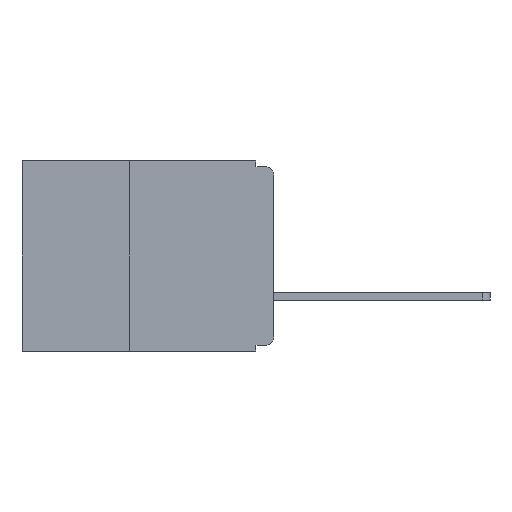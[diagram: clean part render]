
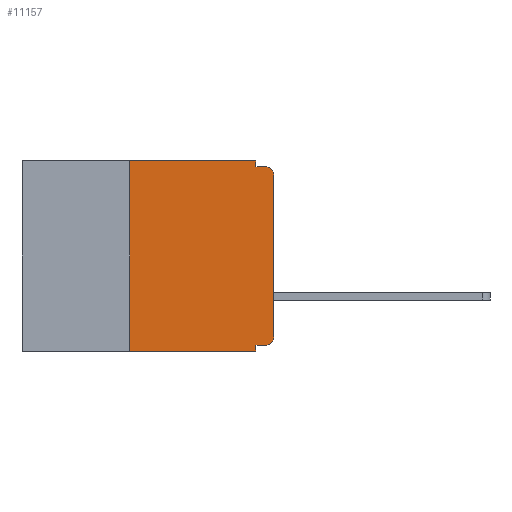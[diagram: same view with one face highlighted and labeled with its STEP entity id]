
A CAD part, left-side view. The second image highlights one B-rep face of the part: STEP entity #11157.
In plain terms, the highlighted planar face has unit normal (-1, 0, 0).
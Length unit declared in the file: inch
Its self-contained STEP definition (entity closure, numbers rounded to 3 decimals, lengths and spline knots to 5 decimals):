
#136 = VECTOR ( 'NONE', #8126, 39.37008 ) ;
#475 = VECTOR ( 'NONE', #18909, 39.37008 ) ;
#684 = EDGE_CURVE ( 'NONE', #23301, #12605, #11262, .T. ) ;
#735 = CARTESIAN_POINT ( 'NONE',  ( 0., 0.015, -0.32 ) ) ;
#1042 = CARTESIAN_POINT ( 'NONE',  ( 0., 0.031, -0.01 ) ) ;
#1107 = LINE ( 'NONE', #12663, #16436 ) ;
#1435 = ORIENTED_EDGE ( 'NONE', *, *, #12381, .F. ) ;
#1779 = ORIENTED_EDGE ( 'NONE', *, *, #684, .F. ) ;
#1916 = VERTEX_POINT ( 'NONE', #17302 ) ;
#2022 = CARTESIAN_POINT ( 'NONE',  ( 0., 0., 0. ) ) ;
#2031 = DIRECTION ( 'NONE',  ( -1., 0., 0. ) ) ;
#2434 = VERTEX_POINT ( 'NONE', #19289 ) ;
#2710 = ORIENTED_EDGE ( 'NONE', *, *, #10901, .F. ) ;
#2767 = EDGE_CURVE ( 'NONE', #20893, #21869, #10214, .T. ) ;
#2868 = DIRECTION ( 'NONE',  ( 0., -1., 0. ) ) ;
#3496 = LINE ( 'NONE', #8178, #4114 ) ;
#3957 = LINE ( 'NONE', #17862, #24506 ) ;
#4114 = VECTOR ( 'NONE', #22052, 39.37008 ) ;
#4262 = ORIENTED_EDGE ( 'NONE', *, *, #14115, .T. ) ;
#4918 = ORIENTED_EDGE ( 'NONE', *, *, #9098, .T. ) ;
#5545 = ORIENTED_EDGE ( 'NONE', *, *, #17180, .T. ) ;
#5755 = DIRECTION ( 'NONE',  ( 1., 0., 0. ) ) ;
#5916 = VECTOR ( 'NONE', #9332, 39.37008 ) ;
#6792 = CARTESIAN_POINT ( 'NONE',  ( 0., 0.031, -0.33 ) ) ;
#7201 = LINE ( 'NONE', #19176, #5916 ) ;
#7562 = EDGE_CURVE ( 'NONE', #19228, #1916, #12766, .T. ) ;
#7900 = CIRCLE ( 'NONE', #21938, 0.015 ) ;
#8126 = DIRECTION ( 'NONE',  ( 0., 0., 1. ) ) ;
#8178 = CARTESIAN_POINT ( 'NONE',  ( 0., 0.437, -0.33 ) ) ;
#9098 = EDGE_CURVE ( 'NONE', #14936, #18371, #7900, .T. ) ;
#9266 = CARTESIAN_POINT ( 'NONE',  ( 0., 0., -0.305 ) ) ;
#9332 = DIRECTION ( 'NONE',  ( 0., 0., 1. ) ) ;
#9596 = CARTESIAN_POINT ( 'NONE',  ( 0., 0.031, -0.32 ) ) ;
#10207 = EDGE_LOOP ( 'NONE', ( #4262, #4918, #2710, #1779, #11879, #25421, #5545, #25133, #1435, #24226 ) ) ;
#10214 = CIRCLE ( 'NONE', #15541, 0.015 ) ;
#10387 = EDGE_CURVE ( 'NONE', #19183, #2434, #7201, .T. ) ;
#10901 = EDGE_CURVE ( 'NONE', #12605, #18371, #15264, .T. ) ;
#11157 = ADVANCED_FACE ( 'NONE', ( #17696 ), #21582, .F. ) ;
#11262 = LINE ( 'NONE', #18875, #475 ) ;
#11639 = CARTESIAN_POINT ( 'NONE',  ( 0., 0.031, 0. ) ) ;
#11763 = DIRECTION ( 'NONE',  ( -1., 0., 0. ) ) ;
#11879 = ORIENTED_EDGE ( 'NONE', *, *, #14281, .F. ) ;
#12354 = CARTESIAN_POINT ( 'NONE',  ( 0., 0.015, -0.305 ) ) ;
#12381 = EDGE_CURVE ( 'NONE', #20893, #19228, #3957, .T. ) ;
#12605 = VERTEX_POINT ( 'NONE', #1042 ) ;
#12663 = CARTESIAN_POINT ( 'NONE',  ( 0., 0.437, 0. ) ) ;
#12766 = LINE ( 'NONE', #6792, #18588 ) ;
#13210 = AXIS2_PLACEMENT_3D ( 'NONE', #17665, #5755, #19660 ) ;
#14039 = CARTESIAN_POINT ( 'NONE',  ( 0., 0.015, -0.025 ) ) ;
#14115 = EDGE_CURVE ( 'NONE', #21869, #14936, #16149, .T. ) ;
#14281 = EDGE_CURVE ( 'NONE', #2434, #23301, #1107, .T. ) ;
#14936 = VERTEX_POINT ( 'NONE', #17018 ) ;
#15264 = LINE ( 'NONE', #18710, #19890 ) ;
#15541 = AXIS2_PLACEMENT_3D ( 'NONE', #12354, #11763, #24618 ) ;
#15979 = DIRECTION ( 'NONE',  ( 0., 1., 0. ) ) ;
#16030 = DIRECTION ( 'NONE',  ( 0., 0., -1. ) ) ;
#16149 = LINE ( 'NONE', #2022, #136 ) ;
#16436 = VECTOR ( 'NONE', #20592, 39.37008 ) ;
#17018 = CARTESIAN_POINT ( 'NONE',  ( 0., 0., -0.025 ) ) ;
#17180 = EDGE_CURVE ( 'NONE', #19183, #1916, #3496, .T. ) ;
#17302 = CARTESIAN_POINT ( 'NONE',  ( 0., 0.031, -0.33 ) ) ;
#17665 = CARTESIAN_POINT ( 'NONE',  ( 0., 0.437, 0. ) ) ;
#17696 = FACE_OUTER_BOUND ( 'NONE', #10207, .T. ) ;
#17862 = CARTESIAN_POINT ( 'NONE',  ( 0., 0., -0.32 ) ) ;
#18371 = VERTEX_POINT ( 'NONE', #24345 ) ;
#18588 = VECTOR ( 'NONE', #22715, 39.37008 ) ;
#18710 = CARTESIAN_POINT ( 'NONE',  ( 0., 0., -0.01 ) ) ;
#18875 = CARTESIAN_POINT ( 'NONE',  ( 0., 0.031, 0. ) ) ;
#18909 = DIRECTION ( 'NONE',  ( 0., 0., -1. ) ) ;
#19176 = CARTESIAN_POINT ( 'NONE',  ( 0., 0.25, -0.33 ) ) ;
#19183 = VERTEX_POINT ( 'NONE', #23284 ) ;
#19228 = VERTEX_POINT ( 'NONE', #9596 ) ;
#19289 = CARTESIAN_POINT ( 'NONE',  ( 0., 0.25, 0. ) ) ;
#19660 = DIRECTION ( 'NONE',  ( 0., 0., -1. ) ) ;
#19890 = VECTOR ( 'NONE', #2868, 39.37008 ) ;
#20592 = DIRECTION ( 'NONE',  ( 0., -1., 0. ) ) ;
#20893 = VERTEX_POINT ( 'NONE', #735 ) ;
#21582 = PLANE ( 'NONE',  #13210 ) ;
#21869 = VERTEX_POINT ( 'NONE', #9266 ) ;
#21938 = AXIS2_PLACEMENT_3D ( 'NONE', #14039, #2031, #16030 ) ;
#22052 = DIRECTION ( 'NONE',  ( 0., -1., 0. ) ) ;
#22715 = DIRECTION ( 'NONE',  ( 0., 0., -1. ) ) ;
#23284 = CARTESIAN_POINT ( 'NONE',  ( 0., 0.25, -0.33 ) ) ;
#23301 = VERTEX_POINT ( 'NONE', #11639 ) ;
#24226 = ORIENTED_EDGE ( 'NONE', *, *, #2767, .T. ) ;
#24345 = CARTESIAN_POINT ( 'NONE',  ( 0., 0.015, -0.01 ) ) ;
#24506 = VECTOR ( 'NONE', #15979, 39.37008 ) ;
#24618 = DIRECTION ( 'NONE',  ( 0., 0., -1. ) ) ;
#25133 = ORIENTED_EDGE ( 'NONE', *, *, #7562, .F. ) ;
#25421 = ORIENTED_EDGE ( 'NONE', *, *, #10387, .F. ) ;
